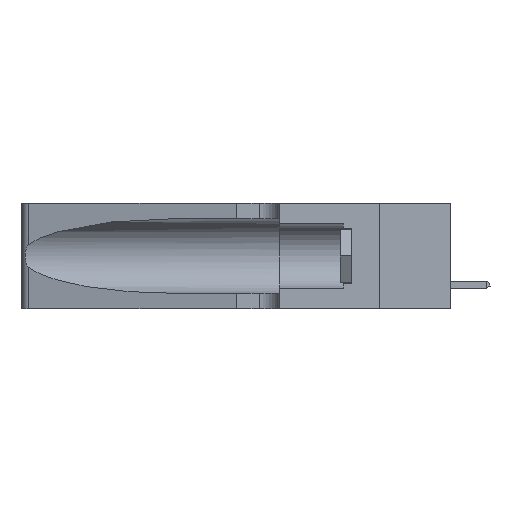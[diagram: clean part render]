
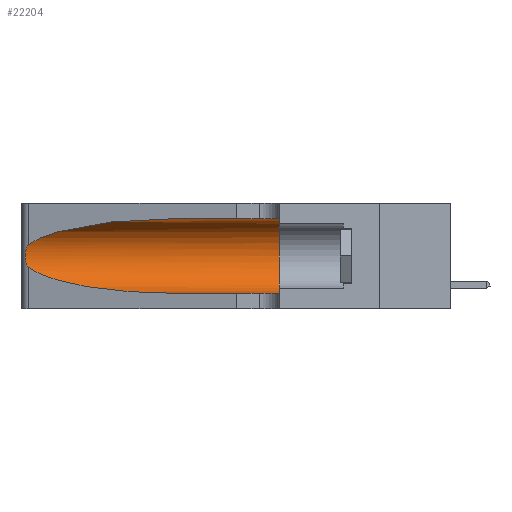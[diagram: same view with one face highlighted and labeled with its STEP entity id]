
A CAD part, left-side view. The second image highlights one B-rep face of the part: STEP entity #22204.
In plain terms, the highlighted cylindrical face has radius 3.308 mm (diameter 6.617 mm), a partial arc.
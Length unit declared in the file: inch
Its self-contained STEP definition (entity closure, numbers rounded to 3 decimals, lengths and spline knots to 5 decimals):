
#561 = DIRECTION ( 'NONE',  ( 0., -1., 0. ) ) ;
#1079 = CARTESIAN_POINT ( 'NONE',  ( 0.25854, 1.2359, 0.20912 ) ) ;
#1257 = CARTESIAN_POINT ( 'NONE',  ( 0.26018, 1.23835, 0.19895 ) ) ;
#1742 = CARTESIAN_POINT ( 'NONE',  ( 0.25787, 1.23484, 0.2124 ) ) ;
#2951 = CARTESIAN_POINT ( 'NONE',  ( 0.1305, 0.72297, 0.31525 ) ) ;
#3130 = EDGE_LOOP ( 'NONE', ( #34376, #36836, #47328, #41968, #36687, #32663 ) ) ;
#3304 = AXIS2_PLACEMENT_3D ( 'NONE', #30374, #45413, #19690 ) ;
#3652 = CYLINDRICAL_SURFACE ( 'NONE', #17848, 0.13025 ) ;
#4279 = CARTESIAN_POINT ( 'NONE',  ( 0.25487, 1.22718, 0.14631 ) ) ;
#4843 = EDGE_CURVE ( 'NONE', #35203, #27999, #20675, .T. ) ;
#6383 = CARTESIAN_POINT ( 'NONE',  ( 0.25487, 1.22718, 0.22369 ) ) ;
#6710 = CARTESIAN_POINT ( 'NONE',  ( 0.2373, 1.15595, 0.28018 ) ) ;
#7148 = DIRECTION ( 'NONE',  ( 0., -1., 0. ) ) ;
#7988 = EDGE_CURVE ( 'NONE', #27042, #28708, #10975, .T. ) ;
#8784 = CARTESIAN_POINT ( 'NONE',  ( 0.25639, 1.23184, 0.21858 ) ) ;
#9260 = CARTESIAN_POINT ( 'NONE',  ( 0.26075, 1.23896, 0.19203 ) ) ;
#9631 = EDGE_CURVE ( 'NONE', #27999, #28708, #32071, .T. ) ;
#10975 = CIRCLE ( 'NONE', #3304, 0.13025 ) ;
#12858 = CARTESIAN_POINT ( 'NONE',  ( 0.26075, 1.23896, 0.178 ) ) ;
#13693 = CARTESIAN_POINT ( 'NONE',  ( 0.2373, 1.15595, 0.08982 ) ) ;
#16782 = EDGE_CURVE ( 'NONE', #33304, #48506, #30293, .T. ) ;
#16839 = CARTESIAN_POINT ( 'NONE',  ( 0.26017, 1.23833, 0.17102 ) ) ;
#17027 = B_SPLINE_CURVE_WITH_KNOTS ( 'NONE', 3,
 ( #41616, #34415, #8784, #1742, #1079, #1257, #9260, #12858, #16839, #27382, #38831, #46514, #35552, #42902 ),
 .UNSPECIFIED., .F., .F.,
 ( 4, 2, 2, 2, 2, 2, 4 ),
 ( 0., 0.00027, 0.00053, 0.00107, 0.0016, 0.00187, 0.00214 ),
 .UNSPECIFIED. ) ;
#17848 = AXIS2_PLACEMENT_3D ( 'NONE', #23260, #561, #26850 ) ;
#17945 = EDGE_CURVE ( 'NONE', #33304, #27042, #40896, .T. ) ;
#18025 = DIRECTION ( 'NONE',  ( 0., -1., 0. ) ) ;
#19690 = DIRECTION ( 'NONE',  ( 0., 0., 1. ) ) ;
#20675 =( BOUNDED_CURVE ( )  B_SPLINE_CURVE ( 3, ( #24400, #13693, #28677, #32109 ),
 .UNSPECIFIED., .F., .T. ) 
 B_SPLINE_CURVE_WITH_KNOTS ( ( 4, 4 ),
 ( 3.44316, 4.71239 ),
 .UNSPECIFIED. ) 
 CURVE ( )  GEOMETRIC_REPRESENTATION_ITEM ( )  RATIONAL_B_SPLINE_CURVE ( ( 1., 0.87, 0.87, 1. ) ) 
 REPRESENTATION_ITEM ( '' )  );
#21222 = CARTESIAN_POINT ( 'NONE',  ( 0.18966, 0.96281, 0.31525 ) ) ;
#21353 = CARTESIAN_POINT ( 'NONE',  ( 0.1305, 1.61858, 0.31525 ) ) ;
#22204 = ADVANCED_FACE ( 'NONE', ( #31838 ), #3652, .F. ) ;
#23260 = CARTESIAN_POINT ( 'NONE',  ( 0.1305, 1.61858, 0.185 ) ) ;
#24400 = CARTESIAN_POINT ( 'NONE',  ( 0.25487, 1.22718, 0.14631 ) ) ;
#26830 = EDGE_CURVE ( 'NONE', #48506, #35203, #17027, .T. ) ;
#26850 = DIRECTION ( 'NONE',  ( 0., 0., -1. ) ) ;
#27042 = VERTEX_POINT ( 'NONE', #36188 ) ;
#27382 = CARTESIAN_POINT ( 'NONE',  ( 0.25856, 1.23593, 0.16098 ) ) ;
#27999 = VERTEX_POINT ( 'NONE', #35214 ) ;
#28677 = CARTESIAN_POINT ( 'NONE',  ( 0.18966, 0.96281, 0.05475 ) ) ;
#28708 = VERTEX_POINT ( 'NONE', #36078 ) ;
#30293 =( BOUNDED_CURVE ( )  B_SPLINE_CURVE ( 3, ( #2951, #21222, #6710, #6383 ),
 .UNSPECIFIED., .F., .T. ) 
 B_SPLINE_CURVE_WITH_KNOTS ( ( 4, 4 ),
 ( 1.5708, 2.84003 ),
 .UNSPECIFIED. ) 
 CURVE ( )  GEOMETRIC_REPRESENTATION_ITEM ( )  RATIONAL_B_SPLINE_CURVE ( ( 1., 0.87, 0.87, 1. ) ) 
 REPRESENTATION_ITEM ( '' )  );
#30374 = CARTESIAN_POINT ( 'NONE',  ( 0.1305, 0.35, 0.185 ) ) ;
#30957 = VECTOR ( 'NONE', #18025, 39.37008 ) ;
#31838 = FACE_OUTER_BOUND ( 'NONE', #3130, .T. ) ;
#32071 = LINE ( 'NONE', #40623, #44945 ) ;
#32109 = CARTESIAN_POINT ( 'NONE',  ( 0.1305, 0.72297, 0.05475 ) ) ;
#32663 = ORIENTED_EDGE ( 'NONE', *, *, #17945, .F. ) ;
#33304 = VERTEX_POINT ( 'NONE', #40895 ) ;
#34376 = ORIENTED_EDGE ( 'NONE', *, *, #16782, .T. ) ;
#34415 = CARTESIAN_POINT ( 'NONE',  ( 0.25555, 1.22994, 0.2215 ) ) ;
#35203 = VERTEX_POINT ( 'NONE', #4279 ) ;
#35214 = CARTESIAN_POINT ( 'NONE',  ( 0.1305, 0.72297, 0.05475 ) ) ;
#35552 = CARTESIAN_POINT ( 'NONE',  ( 0.25555, 1.22993, 0.14849 ) ) ;
#36078 = CARTESIAN_POINT ( 'NONE',  ( 0.1305, 0.35, 0.05475 ) ) ;
#36188 = CARTESIAN_POINT ( 'NONE',  ( 0.1305, 0.35, 0.31525 ) ) ;
#36687 = ORIENTED_EDGE ( 'NONE', *, *, #7988, .F. ) ;
#36836 = ORIENTED_EDGE ( 'NONE', *, *, #26830, .T. ) ;
#38831 = CARTESIAN_POINT ( 'NONE',  ( 0.25789, 1.23486, 0.15765 ) ) ;
#40623 = CARTESIAN_POINT ( 'NONE',  ( 0.1305, 1.61858, 0.05475 ) ) ;
#40895 = CARTESIAN_POINT ( 'NONE',  ( 0.1305, 0.72297, 0.31525 ) ) ;
#40896 = LINE ( 'NONE', #21353, #30957 ) ;
#41616 = CARTESIAN_POINT ( 'NONE',  ( 0.25487, 1.22718, 0.22369 ) ) ;
#41968 = ORIENTED_EDGE ( 'NONE', *, *, #9631, .T. ) ;
#42902 = CARTESIAN_POINT ( 'NONE',  ( 0.25487, 1.22718, 0.14631 ) ) ;
#44945 = VECTOR ( 'NONE', #7148, 39.37008 ) ;
#45413 = DIRECTION ( 'NONE',  ( 0., 1., 0. ) ) ;
#45580 = CARTESIAN_POINT ( 'NONE',  ( 0.25487, 1.22718, 0.22369 ) ) ;
#46514 = CARTESIAN_POINT ( 'NONE',  ( 0.25639, 1.23186, 0.15144 ) ) ;
#47328 = ORIENTED_EDGE ( 'NONE', *, *, #4843, .T. ) ;
#48506 = VERTEX_POINT ( 'NONE', #45580 ) ;
